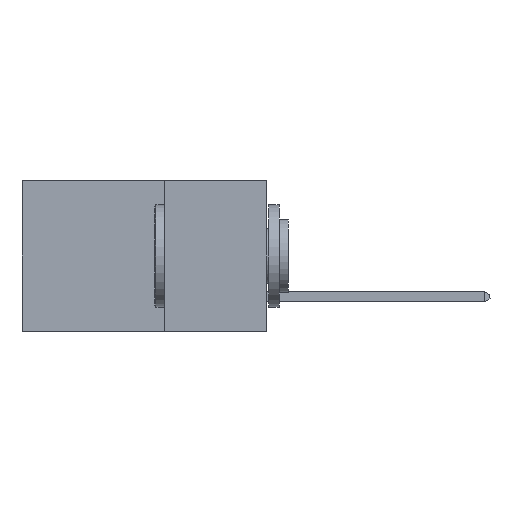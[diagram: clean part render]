
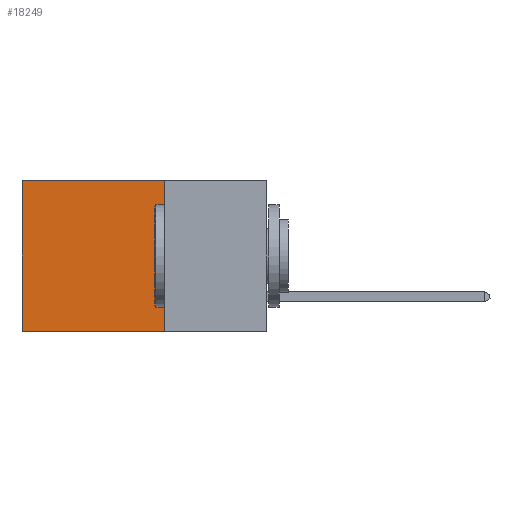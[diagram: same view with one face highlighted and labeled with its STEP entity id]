
A CAD part, left-side view. The second image highlights one B-rep face of the part: STEP entity #18249.
In plain terms, the highlighted planar face has unit normal (-1, 0, 0).
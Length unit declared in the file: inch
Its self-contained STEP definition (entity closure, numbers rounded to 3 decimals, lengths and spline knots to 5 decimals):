
#1098 = EDGE_CURVE ( 'NONE', #28816, #6221, #17435, .T. ) ;
#3182 = LINE ( 'NONE', #3682, #15402 ) ;
#3682 = CARTESIAN_POINT ( 'NONE',  ( 0.2875, 0.25, -0.37 ) ) ;
#4383 = VECTOR ( 'NONE', #17128, 39.37008 ) ;
#4502 = ORIENTED_EDGE ( 'NONE', *, *, #13370, .F. ) ;
#4786 = EDGE_LOOP ( 'NONE', ( #13981, #4502, #16015, #28446 ) ) ;
#5094 = LINE ( 'NONE', #17032, #4383 ) ;
#5680 = VECTOR ( 'NONE', #21392, 39.37008 ) ;
#6221 = VERTEX_POINT ( 'NONE', #22058 ) ;
#6398 = LINE ( 'NONE', #12148, #5680 ) ;
#6886 = VERTEX_POINT ( 'NONE', #15197 ) ;
#7671 = PLANE ( 'NONE',  #19087 ) ;
#11975 = EDGE_CURVE ( 'NONE', #6886, #15793, #5094, .T. ) ;
#12148 = CARTESIAN_POINT ( 'NONE',  ( 0.2875, 0.25, 0. ) ) ;
#12281 = DIRECTION ( 'NONE',  ( 0., 0., -1. ) ) ;
#13370 = EDGE_CURVE ( 'NONE', #15793, #6221, #3182, .T. ) ;
#13981 = ORIENTED_EDGE ( 'NONE', *, *, #1098, .T. ) ;
#15197 = CARTESIAN_POINT ( 'NONE',  ( 0.2875, 0.25, 0. ) ) ;
#15402 = VECTOR ( 'NONE', #19772, 39.37008 ) ;
#15793 = VERTEX_POINT ( 'NONE', #18370 ) ;
#16015 = ORIENTED_EDGE ( 'NONE', *, *, #11975, .F. ) ;
#16713 = VECTOR ( 'NONE', #28380, 39.37008 ) ;
#17032 = CARTESIAN_POINT ( 'NONE',  ( 0.2875, 0.25, 0. ) ) ;
#17128 = DIRECTION ( 'NONE',  ( 0., 0., -1. ) ) ;
#17435 = LINE ( 'NONE', #21433, #16713 ) ;
#18249 = ADVANCED_FACE ( 'NONE', ( #26737 ), #7671, .F. ) ;
#18370 = CARTESIAN_POINT ( 'NONE',  ( 0.2875, 0.25, -0.37 ) ) ;
#19087 = AXIS2_PLACEMENT_3D ( 'NONE', #23741, #26047, #12281 ) ;
#19772 = DIRECTION ( 'NONE',  ( 0., 1., 0. ) ) ;
#20619 = EDGE_CURVE ( 'NONE', #6886, #28816, #6398, .T. ) ;
#21392 = DIRECTION ( 'NONE',  ( 0., 1., 0. ) ) ;
#21433 = CARTESIAN_POINT ( 'NONE',  ( 0.2875, 0.6, 0. ) ) ;
#22058 = CARTESIAN_POINT ( 'NONE',  ( 0.2875, 0.6, -0.37 ) ) ;
#23741 = CARTESIAN_POINT ( 'NONE',  ( 0.2875, 0.25, 0. ) ) ;
#26047 = DIRECTION ( 'NONE',  ( 1., 0., 0. ) ) ;
#26737 = FACE_OUTER_BOUND ( 'NONE', #4786, .T. ) ;
#27142 = CARTESIAN_POINT ( 'NONE',  ( 0.2875, 0.6, 0. ) ) ;
#28380 = DIRECTION ( 'NONE',  ( 0., 0., -1. ) ) ;
#28446 = ORIENTED_EDGE ( 'NONE', *, *, #20619, .T. ) ;
#28816 = VERTEX_POINT ( 'NONE', #27142 ) ;
